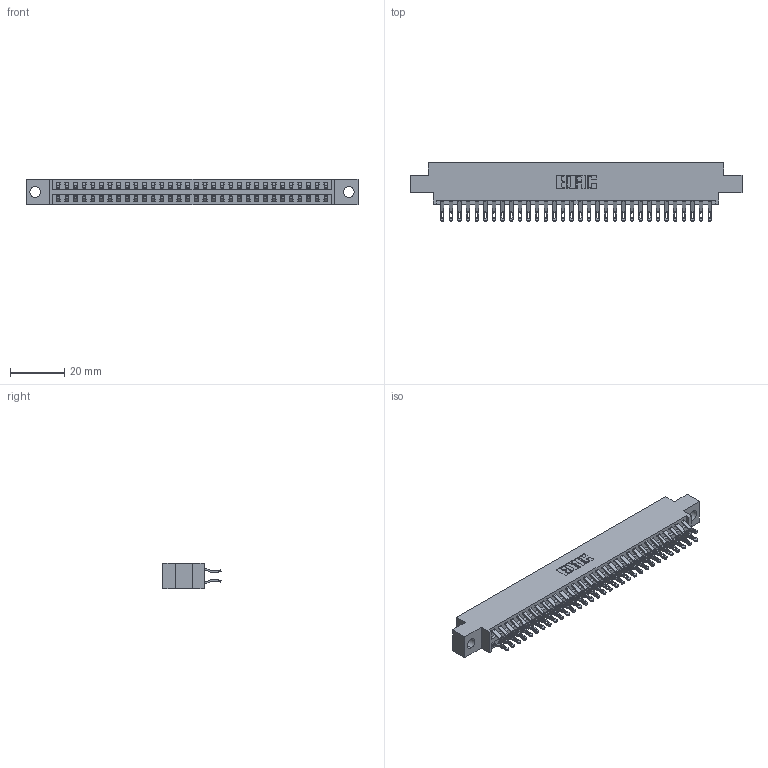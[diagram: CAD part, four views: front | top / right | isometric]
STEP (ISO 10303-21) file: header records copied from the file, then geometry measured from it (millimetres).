
FILE_DESCRIPTION (( 'STEP AP203' ), '1' );
FILE_NAME ('396-064-555-804.STEP', '2018-09-08T17:32:05', ( '' ), ( '' ), 'SwSTEP 2.0', 'SolidWorks 2016', '' );
FILE_SCHEMA (( 'CONFIG_CONTROL_DESIGN' ));
Length unit declared in the file: inch
Products named in the file (3): 346 Part_0.170 Offset - 0.156 Dia-TH; 345-292-001_555 Tail; 396-064-555-804
Assembly tree (65 placements, depth 2):
  396-064-555-804
    346 Part_0.170 Offset - 0.156 Dia-TH
    345-292-001_555 Tail  x64
Bounding box: 122.17 x 21.46 x 9.4 mm (x, y, z)
Volume: 11779 mm3; surface area: 16688.5 mm2
Topology: 65 solids, 65 shells, 3838 faces, 12053 edges, 8034 vertices
Faces by surface type: plane 2192, cylinder 1646
Entity records: 22691 total; most frequent: CARTESIAN_POINT 3790, ORIENTED_EDGE 3694, DIRECTION 3359, EDGE_CURVE 1847, VECTOR 1567, LINE 1567, VERTEX_POINT 1230, AXIS2_PLACEMENT_3D 896
